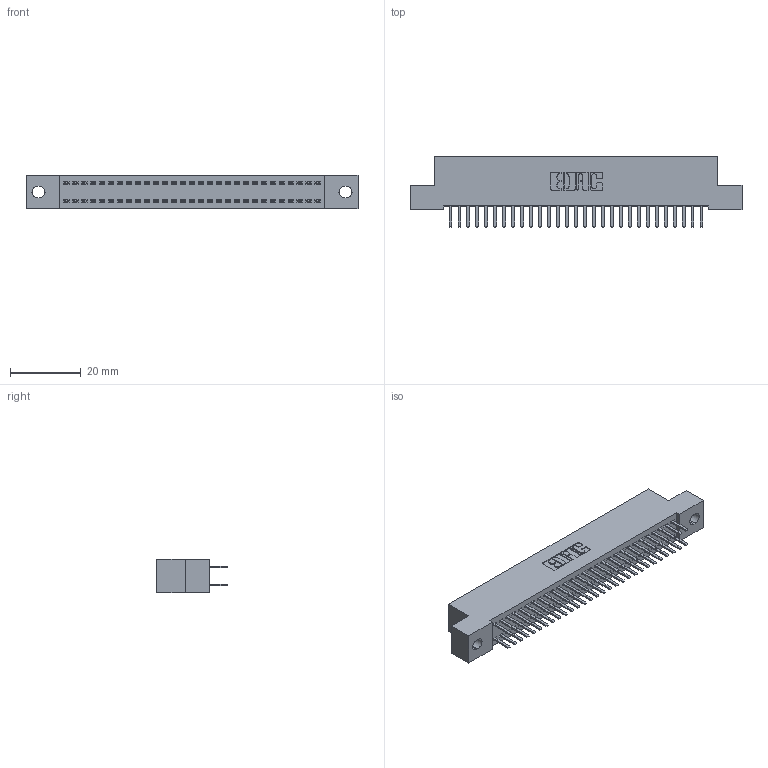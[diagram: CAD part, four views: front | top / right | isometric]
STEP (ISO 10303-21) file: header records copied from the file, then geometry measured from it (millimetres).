
FILE_DESCRIPTION (( 'STEP AP203' ), '1' );
FILE_NAME ('342-058-520-202.STEP', '2019-10-03T12:23:58', ( '' ), ( '' ), 'SwSTEP 2.0', 'SolidWorks 2016', '' );
FILE_SCHEMA (( 'CONFIG_CONTROL_DESIGN' ));
Length unit declared in the file: inch
Products named in the file (3): 342 Part_.128 Slot; 345-292-001_345-293-120; 342-058-520-202
Assembly tree (59 placements, depth 2):
  342-058-520-202
    342 Part_.128 Slot
    345-292-001_345-293-120  x58
Bounding box: 93.98 x 20.02 x 9.4 mm (x, y, z)
Volume: 8304.9 mm3; surface area: 12897.3 mm2
Topology: 59 solids, 59 shells, 3362 faces, 9765 edges, 6354 vertices
Faces by surface type: plane 2274, cylinder 1088
Entity records: 20455 total; most frequent: CARTESIAN_POINT 3418, ORIENTED_EDGE 3342, DIRECTION 2931, EDGE_CURVE 1671, VECTOR 1539, LINE 1539, VERTEX_POINT 1110, AXIS2_PLACEMENT_3D 696
